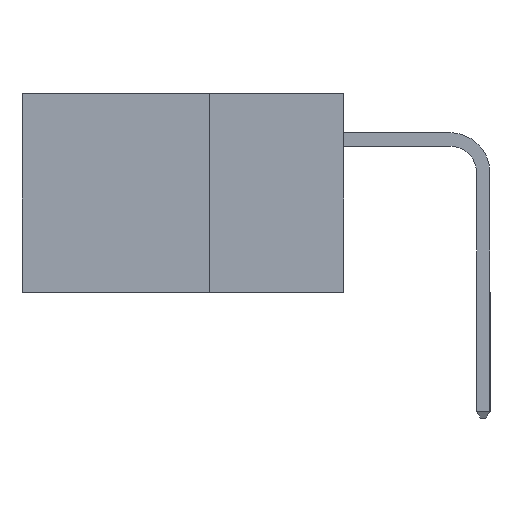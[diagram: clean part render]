
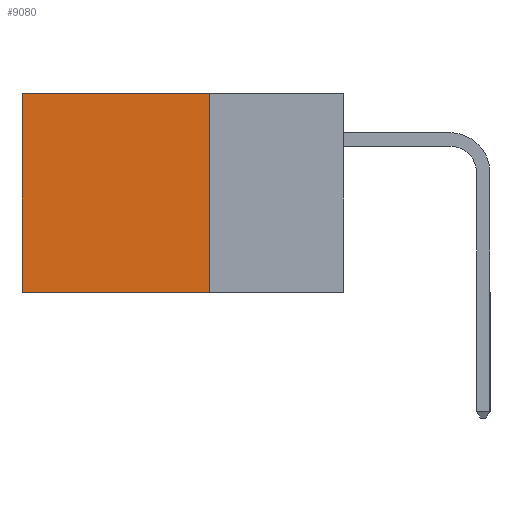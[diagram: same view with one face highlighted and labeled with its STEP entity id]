
A CAD part, left-side view. The second image highlights one B-rep face of the part: STEP entity #9080.
In plain terms, the highlighted planar face has unit normal (-1, 0, 0).
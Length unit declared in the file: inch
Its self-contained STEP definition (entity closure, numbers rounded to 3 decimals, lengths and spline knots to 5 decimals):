
#298 = EDGE_CURVE ( 'NONE', #7198, #2524, #5713, .T. ) ;
#712 = LINE ( 'NONE', #1484, #5190 ) ;
#1072 = ORIENTED_EDGE ( 'NONE', *, *, #298, .T. ) ;
#1484 = CARTESIAN_POINT ( 'NONE',  ( 0.298, 0.6, 0. ) ) ;
#1507 = CARTESIAN_POINT ( 'NONE',  ( 0.298, 0.25, 0. ) ) ;
#1721 = CARTESIAN_POINT ( 'NONE',  ( 0.298, 0.25, 0. ) ) ;
#2229 = EDGE_LOOP ( 'NONE', ( #3338, #8553, #4977, #1072 ) ) ;
#2289 = CARTESIAN_POINT ( 'NONE',  ( 0.298, 0.25, 0. ) ) ;
#2524 = VERTEX_POINT ( 'NONE', #4015 ) ;
#3298 = DIRECTION ( 'NONE',  ( 0., 0., -1. ) ) ;
#3338 = ORIENTED_EDGE ( 'NONE', *, *, #6567, .T. ) ;
#3660 = VERTEX_POINT ( 'NONE', #8370 ) ;
#3878 = DIRECTION ( 'NONE',  ( 0., 1., 0. ) ) ;
#4015 = CARTESIAN_POINT ( 'NONE',  ( 0.298, 0.6, 0. ) ) ;
#4086 = PLANE ( 'NONE',  #7613 ) ;
#4392 = DIRECTION ( 'NONE',  ( 0., 0., -1. ) ) ;
#4548 = LINE ( 'NONE', #5045, #6268 ) ;
#4845 = FACE_OUTER_BOUND ( 'NONE', #2229, .T. ) ;
#4920 = CARTESIAN_POINT ( 'NONE',  ( 0.298, 0.6, -0.37 ) ) ;
#4942 = DIRECTION ( 'NONE',  ( 0., 0., -1. ) ) ;
#4977 = ORIENTED_EDGE ( 'NONE', *, *, #6411, .F. ) ;
#5045 = CARTESIAN_POINT ( 'NONE',  ( 0.298, 0.25, -0.37 ) ) ;
#5062 = LINE ( 'NONE', #1721, #9145 ) ;
#5176 = EDGE_CURVE ( 'NONE', #3660, #8400, #4548, .T. ) ;
#5190 = VECTOR ( 'NONE', #4392, 39.37008 ) ;
#5713 = LINE ( 'NONE', #9643, #6229 ) ;
#6229 = VECTOR ( 'NONE', #9873, 39.37008 ) ;
#6268 = VECTOR ( 'NONE', #3878, 39.37008 ) ;
#6411 = EDGE_CURVE ( 'NONE', #7198, #3660, #5062, .T. ) ;
#6567 = EDGE_CURVE ( 'NONE', #2524, #8400, #712, .T. ) ;
#7198 = VERTEX_POINT ( 'NONE', #1507 ) ;
#7613 = AXIS2_PLACEMENT_3D ( 'NONE', #2289, #9849, #4942 ) ;
#8370 = CARTESIAN_POINT ( 'NONE',  ( 0.298, 0.25, -0.37 ) ) ;
#8400 = VERTEX_POINT ( 'NONE', #4920 ) ;
#8553 = ORIENTED_EDGE ( 'NONE', *, *, #5176, .F. ) ;
#9080 = ADVANCED_FACE ( 'NONE', ( #4845 ), #4086, .F. ) ;
#9145 = VECTOR ( 'NONE', #3298, 39.37008 ) ;
#9643 = CARTESIAN_POINT ( 'NONE',  ( 0.298, 0.25, 0. ) ) ;
#9849 = DIRECTION ( 'NONE',  ( 1., 0., 0. ) ) ;
#9873 = DIRECTION ( 'NONE',  ( 0., 1., 0. ) ) ;
